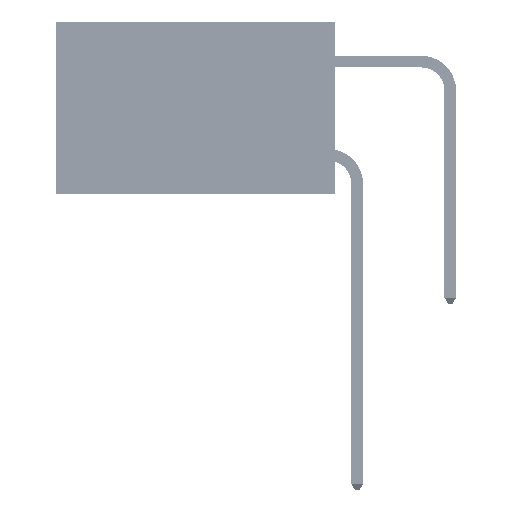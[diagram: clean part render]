
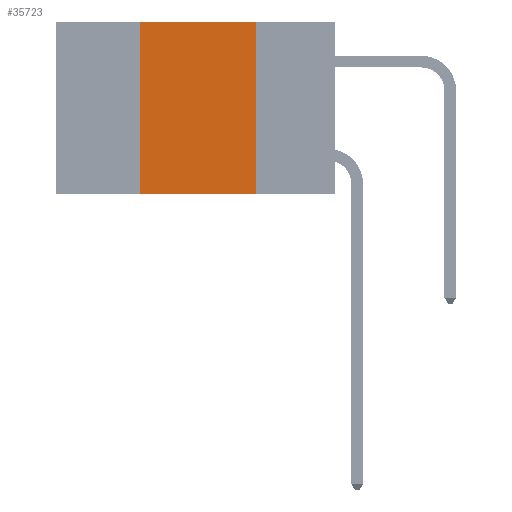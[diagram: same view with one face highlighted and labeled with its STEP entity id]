
A CAD part, left-side view. The second image highlights one B-rep face of the part: STEP entity #35723.
In plain terms, the highlighted planar face has unit normal (-1, 0, 0).
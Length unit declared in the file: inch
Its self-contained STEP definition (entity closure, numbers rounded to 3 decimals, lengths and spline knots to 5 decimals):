
#2983 = DIRECTION ( 'NONE',  ( 0., 0., -1. ) ) ;
#3499 = CARTESIAN_POINT ( 'NONE',  ( 0., 0.17, 0. ) ) ;
#6660 = DIRECTION ( 'NONE',  ( 0., -1., 0. ) ) ;
#7219 = EDGE_LOOP ( 'NONE', ( #7488, #33874, #15912, #13441 ) ) ;
#7488 = ORIENTED_EDGE ( 'NONE', *, *, #38983, .F. ) ;
#10626 = CARTESIAN_POINT ( 'NONE',  ( 0., 0.6, 0. ) ) ;
#12848 = CARTESIAN_POINT ( 'NONE',  ( 0., 0.17, -0.37 ) ) ;
#12906 = FACE_OUTER_BOUND ( 'NONE', #7219, .T. ) ;
#13441 = ORIENTED_EDGE ( 'NONE', *, *, #34151, .T. ) ;
#14286 = CARTESIAN_POINT ( 'NONE',  ( 0., 0.6, -0.37 ) ) ;
#15912 = ORIENTED_EDGE ( 'NONE', *, *, #23494, .F. ) ;
#16873 = PLANE ( 'NONE',  #20405 ) ;
#18940 = VECTOR ( 'NONE', #2983, 39.37008 ) ;
#20405 = AXIS2_PLACEMENT_3D ( 'NONE', #29776, #28995, #21881 ) ;
#21881 = DIRECTION ( 'NONE',  ( 0., 0., -1. ) ) ;
#23494 = EDGE_CURVE ( 'NONE', #45857, #29804, #23644, .T. ) ;
#23551 = LINE ( 'NONE', #10626, #38692 ) ;
#23644 = LINE ( 'NONE', #39754, #41595 ) ;
#25967 = VERTEX_POINT ( 'NONE', #12848 ) ;
#28886 = DIRECTION ( 'NONE',  ( 0., 0., 1. ) ) ;
#28995 = DIRECTION ( 'NONE',  ( 1., 0., 0. ) ) ;
#29776 = CARTESIAN_POINT ( 'NONE',  ( 0., 0.6, 0. ) ) ;
#29804 = VERTEX_POINT ( 'NONE', #41532 ) ;
#31148 = DIRECTION ( 'NONE',  ( 0., -1., 0. ) ) ;
#33874 = ORIENTED_EDGE ( 'NONE', *, *, #48108, .F. ) ;
#34151 = EDGE_CURVE ( 'NONE', #45857, #25967, #43051, .T. ) ;
#35723 = ADVANCED_FACE ( 'NONE', ( #12906 ), #16873, .F. ) ;
#38692 = VECTOR ( 'NONE', #6660, 39.37008 ) ;
#38983 = EDGE_CURVE ( 'NONE', #45423, #25967, #39152, .T. ) ;
#39152 = LINE ( 'NONE', #3499, #18940 ) ;
#39754 = CARTESIAN_POINT ( 'NONE',  ( 0., 0.42, 0. ) ) ;
#41532 = CARTESIAN_POINT ( 'NONE',  ( 0., 0.42, 0. ) ) ;
#41595 = VECTOR ( 'NONE', #28886, 39.37008 ) ;
#43051 = LINE ( 'NONE', #14286, #48154 ) ;
#45423 = VERTEX_POINT ( 'NONE', #47388 ) ;
#45857 = VERTEX_POINT ( 'NONE', #52057 ) ;
#47388 = CARTESIAN_POINT ( 'NONE',  ( 0., 0.17, 0. ) ) ;
#48108 = EDGE_CURVE ( 'NONE', #29804, #45423, #23551, .T. ) ;
#48154 = VECTOR ( 'NONE', #31148, 39.37008 ) ;
#52057 = CARTESIAN_POINT ( 'NONE',  ( 0., 0.42, -0.37 ) ) ;
